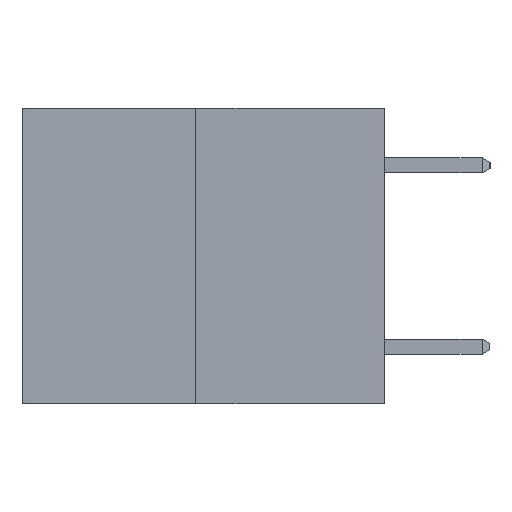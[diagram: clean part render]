
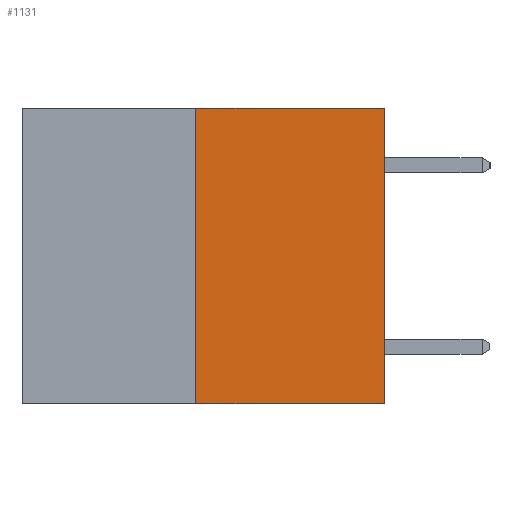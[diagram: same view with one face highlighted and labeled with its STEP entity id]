
A CAD part, left-side view. The second image highlights one B-rep face of the part: STEP entity #1131.
In plain terms, the highlighted planar face has unit normal (-1, 0, 0).
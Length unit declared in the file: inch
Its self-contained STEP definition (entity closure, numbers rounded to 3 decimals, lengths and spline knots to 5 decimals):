
#314 = DIRECTION ( 'NONE',  ( 0., -1., 0. ) ) ;
#525 = EDGE_CURVE ( 'NONE', #7713, #3610, #11423, .T. ) ;
#877 = DIRECTION ( 'NONE',  ( 0., 0., 1. ) ) ;
#1082 = CARTESIAN_POINT ( 'NONE',  ( 0., 0.6, 0. ) ) ;
#1131 = ADVANCED_FACE ( 'NONE', ( #7341 ), #7553, .F. ) ;
#1618 = ORIENTED_EDGE ( 'NONE', *, *, #525, .F. ) ;
#2106 = DIRECTION ( 'NONE',  ( 1., 0., 0. ) ) ;
#2426 = ORIENTED_EDGE ( 'NONE', *, *, #2544, .T. ) ;
#2469 = LINE ( 'NONE', #6747, #3581 ) ;
#2534 = CARTESIAN_POINT ( 'NONE',  ( 0., 0.6, -0.49 ) ) ;
#2544 = EDGE_CURVE ( 'NONE', #11602, #3610, #2469, .T. ) ;
#2728 = ORIENTED_EDGE ( 'NONE', *, *, #5940, .F. ) ;
#3581 = VECTOR ( 'NONE', #6696, 39.37008 ) ;
#3610 = VERTEX_POINT ( 'NONE', #4097 ) ;
#4097 = CARTESIAN_POINT ( 'NONE',  ( 0., 0., 0. ) ) ;
#4666 = AXIS2_PLACEMENT_3D ( 'NONE', #1082, #2106, #8513 ) ;
#5721 = CARTESIAN_POINT ( 'NONE',  ( 0., 0., -0.49 ) ) ;
#5940 = EDGE_CURVE ( 'NONE', #9047, #7713, #9375, .T. ) ;
#6313 = LINE ( 'NONE', #2534, #7766 ) ;
#6696 = DIRECTION ( 'NONE',  ( 0., 0., 1. ) ) ;
#6747 = CARTESIAN_POINT ( 'NONE',  ( 0., 0., 0. ) ) ;
#6960 = VECTOR ( 'NONE', #877, 39.37008 ) ;
#7341 = FACE_OUTER_BOUND ( 'NONE', #11669, .T. ) ;
#7553 = PLANE ( 'NONE',  #4666 ) ;
#7713 = VERTEX_POINT ( 'NONE', #11287 ) ;
#7766 = VECTOR ( 'NONE', #11744, 39.37008 ) ;
#8074 = CARTESIAN_POINT ( 'NONE',  ( 0., 0.312, -0.49 ) ) ;
#8513 = DIRECTION ( 'NONE',  ( 0., 0., -1. ) ) ;
#9047 = VERTEX_POINT ( 'NONE', #8074 ) ;
#9375 = LINE ( 'NONE', #11696, #6960 ) ;
#9486 = CARTESIAN_POINT ( 'NONE',  ( 0., 0.6, 0. ) ) ;
#9555 = EDGE_CURVE ( 'NONE', #9047, #11602, #6313, .T. ) ;
#10727 = VECTOR ( 'NONE', #314, 39.37008 ) ;
#11023 = ORIENTED_EDGE ( 'NONE', *, *, #9555, .T. ) ;
#11287 = CARTESIAN_POINT ( 'NONE',  ( 0., 0.312, 0. ) ) ;
#11423 = LINE ( 'NONE', #9486, #10727 ) ;
#11602 = VERTEX_POINT ( 'NONE', #5721 ) ;
#11669 = EDGE_LOOP ( 'NONE', ( #2728, #11023, #2426, #1618 ) ) ;
#11696 = CARTESIAN_POINT ( 'NONE',  ( 0., 0.312, -0.49 ) ) ;
#11744 = DIRECTION ( 'NONE',  ( 0., -1., 0. ) ) ;
